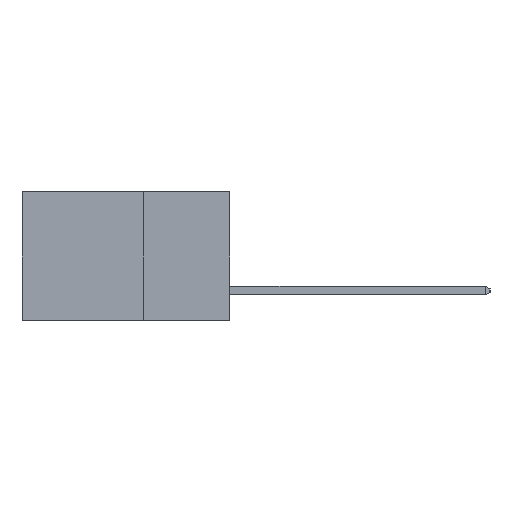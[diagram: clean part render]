
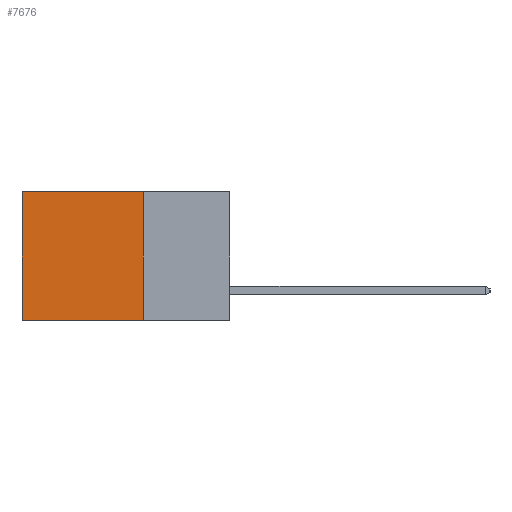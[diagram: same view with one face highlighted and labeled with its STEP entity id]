
A CAD part, left-side view. The second image highlights one B-rep face of the part: STEP entity #7676.
In plain terms, the highlighted planar face has unit normal (-1, 0, 0).
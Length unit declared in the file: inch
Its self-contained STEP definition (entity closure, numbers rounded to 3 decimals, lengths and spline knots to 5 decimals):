
#525 = ORIENTED_EDGE ( 'NONE', *, *, #4596, .T. ) ;
#860 = VERTEX_POINT ( 'NONE', #10789 ) ;
#913 = DIRECTION ( 'NONE',  ( 0., 0., -1. ) ) ;
#963 = CARTESIAN_POINT ( 'NONE',  ( 0.2615, 0.25, -0.37 ) ) ;
#1367 = VECTOR ( 'NONE', #5331, 39.37008 ) ;
#1731 = CARTESIAN_POINT ( 'NONE',  ( 0.2615, 0.6, -0.37 ) ) ;
#2705 = CARTESIAN_POINT ( 'NONE',  ( 0.2615, 0.25, 0. ) ) ;
#2812 = DIRECTION ( 'NONE',  ( 1., 0., 0. ) ) ;
#3421 = CARTESIAN_POINT ( 'NONE',  ( 0.2615, 0.25, -0.37 ) ) ;
#3526 = DIRECTION ( 'NONE',  ( 0., 1., 0. ) ) ;
#3555 = VERTEX_POINT ( 'NONE', #2705 ) ;
#4003 = LINE ( 'NONE', #1731, #8188 ) ;
#4209 = FACE_OUTER_BOUND ( 'NONE', #10788, .T. ) ;
#4265 = AXIS2_PLACEMENT_3D ( 'NONE', #7877, #2812, #8704 ) ;
#4596 = EDGE_CURVE ( 'NONE', #3555, #10195, #6399, .T. ) ;
#4683 = EDGE_CURVE ( 'NONE', #860, #4814, #4839, .T. ) ;
#4814 = VERTEX_POINT ( 'NONE', #10298 ) ;
#4839 = LINE ( 'NONE', #3421, #9969 ) ;
#5145 = CARTESIAN_POINT ( 'NONE',  ( 0.2615, 0.6, 0. ) ) ;
#5331 = DIRECTION ( 'NONE',  ( 0., 1., 0. ) ) ;
#5339 = CARTESIAN_POINT ( 'NONE',  ( 0.2615, 0.25, 0. ) ) ;
#5382 = PLANE ( 'NONE',  #4265 ) ;
#5711 = ORIENTED_EDGE ( 'NONE', *, *, #4683, .F. ) ;
#6150 = LINE ( 'NONE', #963, #8351 ) ;
#6300 = EDGE_CURVE ( 'NONE', #10195, #4814, #4003, .T. ) ;
#6368 = ORIENTED_EDGE ( 'NONE', *, *, #6300, .T. ) ;
#6399 = LINE ( 'NONE', #5339, #1367 ) ;
#6857 = DIRECTION ( 'NONE',  ( 0., 0., -1. ) ) ;
#7676 = ADVANCED_FACE ( 'NONE', ( #4209 ), #5382, .F. ) ;
#7877 = CARTESIAN_POINT ( 'NONE',  ( 0.2615, 0.25, -0.37 ) ) ;
#8188 = VECTOR ( 'NONE', #913, 39.37008 ) ;
#8351 = VECTOR ( 'NONE', #6857, 39.37008 ) ;
#8704 = DIRECTION ( 'NONE',  ( 0., 0., -1. ) ) ;
#8981 = EDGE_CURVE ( 'NONE', #3555, #860, #6150, .T. ) ;
#9262 = ORIENTED_EDGE ( 'NONE', *, *, #8981, .F. ) ;
#9969 = VECTOR ( 'NONE', #3526, 39.37008 ) ;
#10195 = VERTEX_POINT ( 'NONE', #5145 ) ;
#10298 = CARTESIAN_POINT ( 'NONE',  ( 0.2615, 0.6, -0.37 ) ) ;
#10788 = EDGE_LOOP ( 'NONE', ( #6368, #5711, #9262, #525 ) ) ;
#10789 = CARTESIAN_POINT ( 'NONE',  ( 0.2615, 0.25, -0.37 ) ) ;
